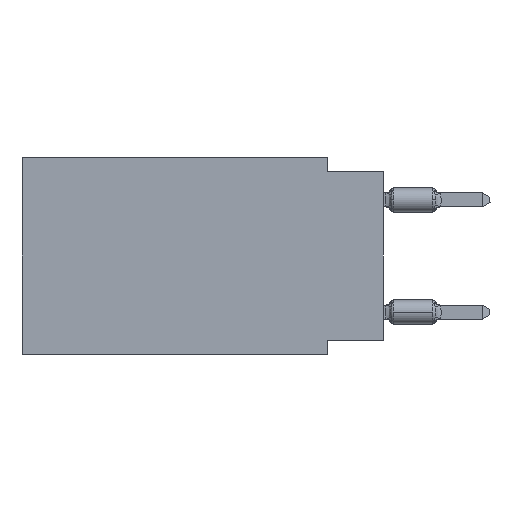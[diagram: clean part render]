
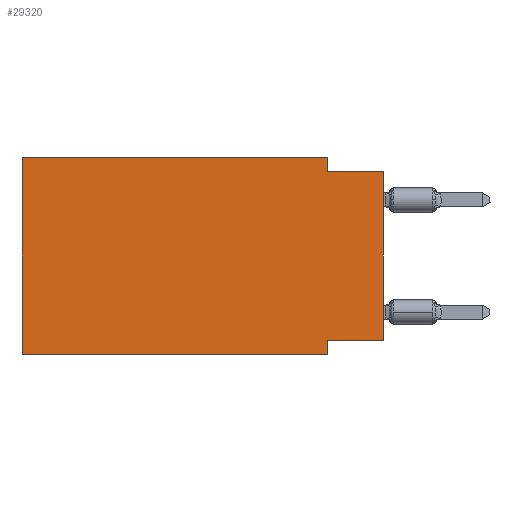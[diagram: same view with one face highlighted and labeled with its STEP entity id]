
A CAD part, left-side view. The second image highlights one B-rep face of the part: STEP entity #29320.
In plain terms, the highlighted planar face has unit normal (-1, 0, 0).
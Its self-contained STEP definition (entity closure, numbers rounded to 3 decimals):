
#159 = CARTESIAN_POINT ( 'NONE',  ( 0., 2.54, 0. ) ) ;
#2335 = DIRECTION ( 'NONE',  ( 0., 0., -1. ) ) ;
#4646 = ORIENTED_EDGE ( 'NONE', *, *, #5308, .F. ) ;
#5308 = EDGE_CURVE ( 'NONE', #39510, #47803, #47618, .T. ) ;
#5628 = EDGE_LOOP ( 'NONE', ( #14926, #34264, #47267, #39638, #44416, #7839, #4646, #29512 ) ) ;
#5871 = CARTESIAN_POINT ( 'NONE',  ( 0., 16.383, -8.89 ) ) ;
#6366 = VECTOR ( 'NONE', #22424, 1000. ) ;
#6804 = AXIS2_PLACEMENT_3D ( 'NONE', #53029, #43086, #48348 ) ;
#6841 = CARTESIAN_POINT ( 'NONE',  ( 0., 16.383, 0. ) ) ;
#7127 = LINE ( 'NONE', #6841, #24803 ) ;
#7839 = ORIENTED_EDGE ( 'NONE', *, *, #56708, .T. ) ;
#8293 = VECTOR ( 'NONE', #42953, 1000. ) ;
#11108 = CARTESIAN_POINT ( 'NONE',  ( 0., 16.383, 0. ) ) ;
#11742 = VECTOR ( 'NONE', #43797, 1000. ) ;
#12045 = VERTEX_POINT ( 'NONE', #43983 ) ;
#12435 = VECTOR ( 'NONE', #2335, 1000. ) ;
#13094 = VECTOR ( 'NONE', #37712, 1000. ) ;
#14926 = ORIENTED_EDGE ( 'NONE', *, *, #16731, .T. ) ;
#16031 = LINE ( 'NONE', #33875, #8293 ) ;
#16731 = EDGE_CURVE ( 'NONE', #46917, #31877, #53464, .T. ) ;
#17015 = CARTESIAN_POINT ( 'NONE',  ( 0., 2.54, -8.89 ) ) ;
#19894 = CARTESIAN_POINT ( 'NONE',  ( 0., 16.383, -8.89 ) ) ;
#20429 = CARTESIAN_POINT ( 'NONE',  ( 0., 2.54, -0.635 ) ) ;
#22424 = DIRECTION ( 'NONE',  ( 0., 0., 1. ) ) ;
#24352 = VERTEX_POINT ( 'NONE', #5871 ) ;
#24803 = VECTOR ( 'NONE', #46649, 1000. ) ;
#28949 = LINE ( 'NONE', #42986, #13094 ) ;
#29320 = ADVANCED_FACE ( 'NONE', ( #38107 ), #55972, .F. ) ;
#29512 = ORIENTED_EDGE ( 'NONE', *, *, #49992, .F. ) ;
#29932 = EDGE_CURVE ( 'NONE', #39613, #45593, #56184, .T. ) ;
#31877 = VERTEX_POINT ( 'NONE', #55022 ) ;
#33875 = CARTESIAN_POINT ( 'NONE',  ( 0., 0., -8.255 ) ) ;
#34213 = CARTESIAN_POINT ( 'NONE',  ( 0., 2.54, 0. ) ) ;
#34264 = ORIENTED_EDGE ( 'NONE', *, *, #37066, .F. ) ;
#35361 = EDGE_CURVE ( 'NONE', #12045, #39613, #51204, .T. ) ;
#36140 = CARTESIAN_POINT ( 'NONE',  ( 0., 0., -8.255 ) ) ;
#37066 = EDGE_CURVE ( 'NONE', #45593, #31877, #28949, .T. ) ;
#37712 = DIRECTION ( 'NONE',  ( 0., -1., 0. ) ) ;
#38107 = FACE_OUTER_BOUND ( 'NONE', #5628, .T. ) ;
#38322 = LINE ( 'NONE', #19894, #50209 ) ;
#39510 = VERTEX_POINT ( 'NONE', #42604 ) ;
#39613 = VERTEX_POINT ( 'NONE', #159 ) ;
#39638 = ORIENTED_EDGE ( 'NONE', *, *, #35361, .F. ) ;
#42604 = CARTESIAN_POINT ( 'NONE',  ( 0., 2.54, -8.255 ) ) ;
#42953 = DIRECTION ( 'NONE',  ( 0., 1., 0. ) ) ;
#42986 = CARTESIAN_POINT ( 'NONE',  ( 0., 0., -0.635 ) ) ;
#43086 = DIRECTION ( 'NONE',  ( 1., 0., 0. ) ) ;
#43221 = CARTESIAN_POINT ( 'NONE',  ( 0., 2.54, -8.89 ) ) ;
#43338 = EDGE_CURVE ( 'NONE', #24352, #12045, #7127, .T. ) ;
#43797 = DIRECTION ( 'NONE',  ( 0., 0., -1. ) ) ;
#43983 = CARTESIAN_POINT ( 'NONE',  ( 0., 16.383, 0. ) ) ;
#44416 = ORIENTED_EDGE ( 'NONE', *, *, #43338, .F. ) ;
#45593 = VERTEX_POINT ( 'NONE', #20429 ) ;
#46649 = DIRECTION ( 'NONE',  ( 0., 0., 1. ) ) ;
#46819 = DIRECTION ( 'NONE',  ( 0., -1., 0. ) ) ;
#46838 = DIRECTION ( 'NONE',  ( 0., -1., 0. ) ) ;
#46917 = VERTEX_POINT ( 'NONE', #36140 ) ;
#47267 = ORIENTED_EDGE ( 'NONE', *, *, #29932, .F. ) ;
#47618 = LINE ( 'NONE', #43221, #11742 ) ;
#47803 = VERTEX_POINT ( 'NONE', #17015 ) ;
#48348 = DIRECTION ( 'NONE',  ( 0., 0., -1. ) ) ;
#49992 = EDGE_CURVE ( 'NONE', #46917, #39510, #16031, .T. ) ;
#50209 = VECTOR ( 'NONE', #46838, 1000. ) ;
#51204 = LINE ( 'NONE', #11108, #52212 ) ;
#52212 = VECTOR ( 'NONE', #46819, 1000. ) ;
#53029 = CARTESIAN_POINT ( 'NONE',  ( 0., 16.383, 0. ) ) ;
#53464 = LINE ( 'NONE', #57277, #6366 ) ;
#55022 = CARTESIAN_POINT ( 'NONE',  ( 0., 0., -0.635 ) ) ;
#55972 = PLANE ( 'NONE',  #6804 ) ;
#56184 = LINE ( 'NONE', #34213, #12435 ) ;
#56708 = EDGE_CURVE ( 'NONE', #24352, #47803, #38322, .T. ) ;
#57277 = CARTESIAN_POINT ( 'NONE',  ( 0., 0., 0. ) ) ;
